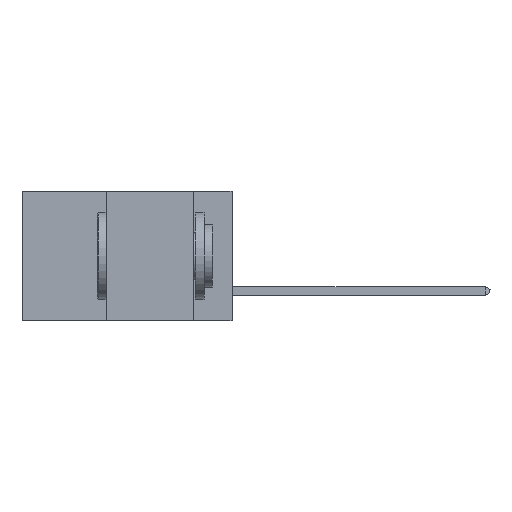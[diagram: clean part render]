
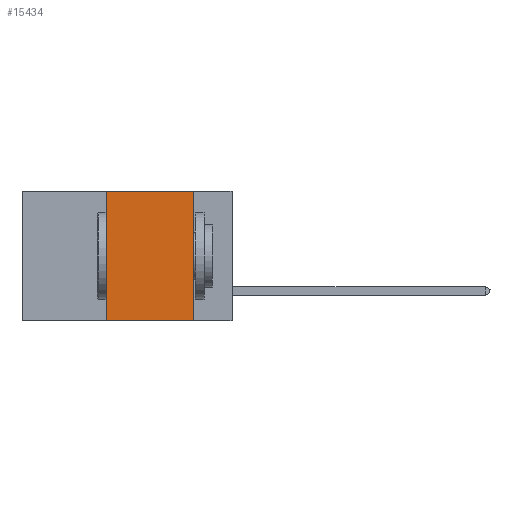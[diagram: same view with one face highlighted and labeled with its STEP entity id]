
A CAD part, left-side view. The second image highlights one B-rep face of the part: STEP entity #15434.
In plain terms, the highlighted planar face has unit normal (-1, 0, 0).
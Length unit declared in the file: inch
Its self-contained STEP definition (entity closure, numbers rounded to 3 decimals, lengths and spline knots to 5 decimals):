
#218 = ORIENTED_EDGE ( 'NONE', *, *, #12652, .T. ) ;
#565 = DIRECTION ( 'NONE',  ( 0., 0., -1. ) ) ;
#995 = ORIENTED_EDGE ( 'NONE', *, *, #14774, .F. ) ;
#1239 = VECTOR ( 'NONE', #7520, 39.37008 ) ;
#2218 = CARTESIAN_POINT ( 'NONE',  ( 0., 0.11, 0. ) ) ;
#2434 = VERTEX_POINT ( 'NONE', #9804 ) ;
#3704 = DIRECTION ( 'NONE',  ( 0., -1., 0. ) ) ;
#3752 = VERTEX_POINT ( 'NONE', #7440 ) ;
#3833 = AXIS2_PLACEMENT_3D ( 'NONE', #15256, #16616, #565 ) ;
#4066 = LINE ( 'NONE', #5135, #9553 ) ;
#5135 = CARTESIAN_POINT ( 'NONE',  ( 0., 0.6, 0. ) ) ;
#5790 = VECTOR ( 'NONE', #7564, 39.37008 ) ;
#6071 = LINE ( 'NONE', #14146, #12198 ) ;
#7080 = PLANE ( 'NONE',  #3833 ) ;
#7440 = CARTESIAN_POINT ( 'NONE',  ( 0., 0.11, -0.37 ) ) ;
#7520 = DIRECTION ( 'NONE',  ( 0., 0., 1. ) ) ;
#7564 = DIRECTION ( 'NONE',  ( 0., 0., -1. ) ) ;
#7766 = ORIENTED_EDGE ( 'NONE', *, *, #11521, .F. ) ;
#9553 = VECTOR ( 'NONE', #3704, 39.37008 ) ;
#9804 = CARTESIAN_POINT ( 'NONE',  ( 0., 0.36, 0. ) ) ;
#10294 = CARTESIAN_POINT ( 'NONE',  ( 0., 0.36, 0. ) ) ;
#11493 = LINE ( 'NONE', #2218, #5790 ) ;
#11521 = EDGE_CURVE ( 'NONE', #2434, #13225, #4066, .T. ) ;
#11799 = CARTESIAN_POINT ( 'NONE',  ( 0., 0.36, -0.37 ) ) ;
#11926 = FACE_OUTER_BOUND ( 'NONE', #13905, .T. ) ;
#12102 = LINE ( 'NONE', #10294, #1239 ) ;
#12198 = VECTOR ( 'NONE', #15516, 39.37008 ) ;
#12652 = EDGE_CURVE ( 'NONE', #13511, #3752, #6071, .T. ) ;
#13225 = VERTEX_POINT ( 'NONE', #17144 ) ;
#13511 = VERTEX_POINT ( 'NONE', #11799 ) ;
#13905 = EDGE_LOOP ( 'NONE', ( #995, #7766, #16183, #218 ) ) ;
#14146 = CARTESIAN_POINT ( 'NONE',  ( 0., 0.6, -0.37 ) ) ;
#14774 = EDGE_CURVE ( 'NONE', #13225, #3752, #11493, .T. ) ;
#15256 = CARTESIAN_POINT ( 'NONE',  ( 0., 0.6, 0. ) ) ;
#15434 = ADVANCED_FACE ( 'NONE', ( #11926 ), #7080, .F. ) ;
#15516 = DIRECTION ( 'NONE',  ( 0., -1., 0. ) ) ;
#16043 = EDGE_CURVE ( 'NONE', #13511, #2434, #12102, .T. ) ;
#16183 = ORIENTED_EDGE ( 'NONE', *, *, #16043, .F. ) ;
#16616 = DIRECTION ( 'NONE',  ( 1., 0., 0. ) ) ;
#17144 = CARTESIAN_POINT ( 'NONE',  ( 0., 0.11, 0. ) ) ;
